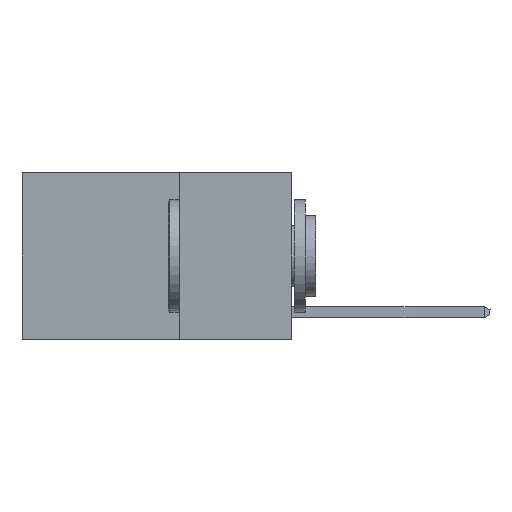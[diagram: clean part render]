
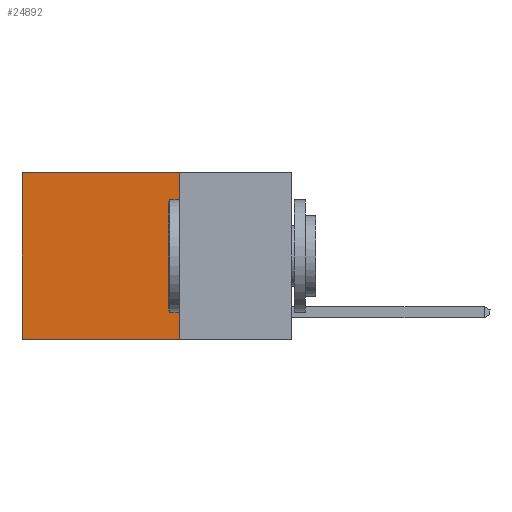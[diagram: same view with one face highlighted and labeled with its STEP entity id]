
A CAD part, left-side view. The second image highlights one B-rep face of the part: STEP entity #24892.
In plain terms, the highlighted planar face has unit normal (-1, 0, 0).
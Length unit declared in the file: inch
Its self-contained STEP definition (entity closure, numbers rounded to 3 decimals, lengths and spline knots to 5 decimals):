
#216 = CARTESIAN_POINT ( 'NONE',  ( 0.2625, 0.25, -0.37 ) ) ;
#452 = VECTOR ( 'NONE', #13915, 39.37008 ) ;
#1127 = ORIENTED_EDGE ( 'NONE', *, *, #7266, .T. ) ;
#1210 = CARTESIAN_POINT ( 'NONE',  ( 0.2625, 0.6, 0. ) ) ;
#3529 = LINE ( 'NONE', #216, #9721 ) ;
#3924 = CARTESIAN_POINT ( 'NONE',  ( 0.2625, 0.25, 0. ) ) ;
#4786 = FACE_OUTER_BOUND ( 'NONE', #11302, .T. ) ;
#5163 = LINE ( 'NONE', #10801, #25716 ) ;
#5876 = EDGE_CURVE ( 'NONE', #10140, #17563, #5163, .T. ) ;
#7146 = EDGE_CURVE ( 'NONE', #14855, #9823, #18463, .T. ) ;
#7266 = EDGE_CURVE ( 'NONE', #10140, #14855, #8841, .T. ) ;
#7859 = CARTESIAN_POINT ( 'NONE',  ( 0.2625, 0.25, 0. ) ) ;
#8841 = LINE ( 'NONE', #7859, #452 ) ;
#9721 = VECTOR ( 'NONE', #18014, 39.37008 ) ;
#9823 = VERTEX_POINT ( 'NONE', #16643 ) ;
#10140 = VERTEX_POINT ( 'NONE', #3924 ) ;
#10801 = CARTESIAN_POINT ( 'NONE',  ( 0.2625, 0.25, 0. ) ) ;
#11302 = EDGE_LOOP ( 'NONE', ( #15982, #19259, #18272, #1127 ) ) ;
#12787 = DIRECTION ( 'NONE',  ( 0., 0., -1. ) ) ;
#13468 = EDGE_CURVE ( 'NONE', #17563, #9823, #3529, .T. ) ;
#13747 = CARTESIAN_POINT ( 'NONE',  ( 0.2625, 0.25, 0. ) ) ;
#13915 = DIRECTION ( 'NONE',  ( 0., 1., 0. ) ) ;
#14808 = CARTESIAN_POINT ( 'NONE',  ( 0.2625, 0.6, 0. ) ) ;
#14855 = VERTEX_POINT ( 'NONE', #14808 ) ;
#15041 = VECTOR ( 'NONE', #19094, 39.37008 ) ;
#15434 = DIRECTION ( 'NONE',  ( 0., 0., -1. ) ) ;
#15589 = DIRECTION ( 'NONE',  ( 1., 0., 0. ) ) ;
#15855 = CARTESIAN_POINT ( 'NONE',  ( 0.2625, 0.25, -0.37 ) ) ;
#15982 = ORIENTED_EDGE ( 'NONE', *, *, #7146, .T. ) ;
#16643 = CARTESIAN_POINT ( 'NONE',  ( 0.2625, 0.6, -0.37 ) ) ;
#17563 = VERTEX_POINT ( 'NONE', #15855 ) ;
#18014 = DIRECTION ( 'NONE',  ( 0., 1., 0. ) ) ;
#18272 = ORIENTED_EDGE ( 'NONE', *, *, #5876, .F. ) ;
#18463 = LINE ( 'NONE', #1210, #15041 ) ;
#19094 = DIRECTION ( 'NONE',  ( 0., 0., -1. ) ) ;
#19259 = ORIENTED_EDGE ( 'NONE', *, *, #13468, .F. ) ;
#21195 = AXIS2_PLACEMENT_3D ( 'NONE', #13747, #15589, #15434 ) ;
#23354 = PLANE ( 'NONE',  #21195 ) ;
#24892 = ADVANCED_FACE ( 'NONE', ( #4786 ), #23354, .F. ) ;
#25716 = VECTOR ( 'NONE', #12787, 39.37008 ) ;
